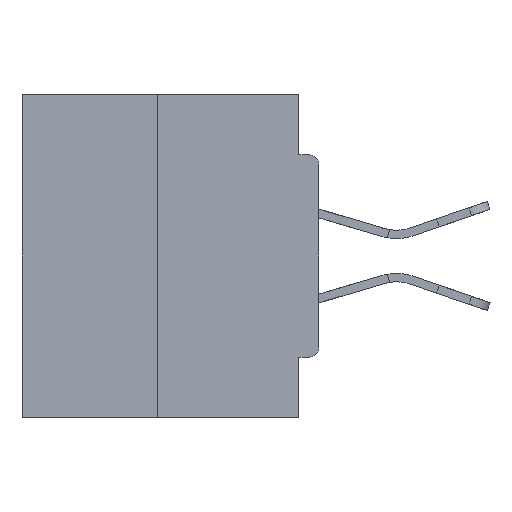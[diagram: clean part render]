
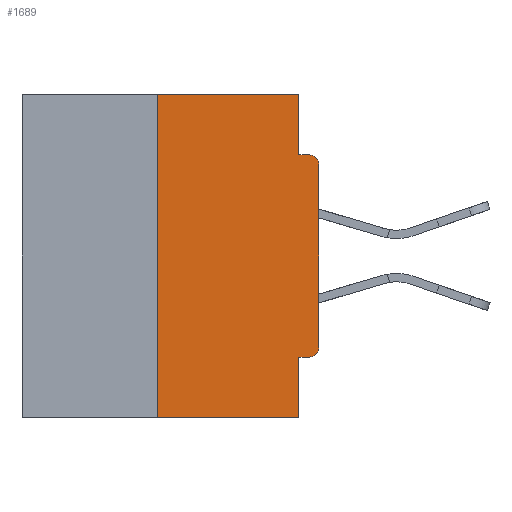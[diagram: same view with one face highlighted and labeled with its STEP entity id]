
A CAD part, left-side view. The second image highlights one B-rep face of the part: STEP entity #1689.
In plain terms, the highlighted planar face has unit normal (-1, 0, 0).
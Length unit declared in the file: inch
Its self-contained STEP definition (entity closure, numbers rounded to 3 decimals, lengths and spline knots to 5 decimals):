
#196 = CARTESIAN_POINT ( 'NONE',  ( 0., 0.031, 0. ) ) ;
#494 = DIRECTION ( 'NONE',  ( 0., 0., 1. ) ) ;
#618 = LINE ( 'NONE', #21622, #19033 ) ;
#691 = VECTOR ( 'NONE', #16077, 39.37008 ) ;
#942 = VERTEX_POINT ( 'NONE', #22931 ) ;
#1689 = ADVANCED_FACE ( 'NONE', ( #21442 ), #31949, .F. ) ;
#1726 = LINE ( 'NONE', #17066, #4128 ) ;
#1765 = AXIS2_PLACEMENT_3D ( 'NONE', #20414, #2351, #12517 ) ;
#2313 = LINE ( 'NONE', #7808, #17178 ) ;
#2351 = DIRECTION ( 'NONE',  ( -1., 0., 0. ) ) ;
#2788 = CARTESIAN_POINT ( 'NONE',  ( 0., 0.015, -0.1085 ) ) ;
#3073 = LINE ( 'NONE', #11176, #21508 ) ;
#3281 = ORIENTED_EDGE ( 'NONE', *, *, #24831, .F. ) ;
#3482 = EDGE_LOOP ( 'NONE', ( #13902, #20780, #18698, #6443, #3281, #6612, #5165, #19650, #14444, #18623 ) ) ;
#3980 = CIRCLE ( 'NONE', #1765, 0.015 ) ;
#4121 = AXIS2_PLACEMENT_3D ( 'NONE', #23693, #24210, #31613 ) ;
#4128 = VECTOR ( 'NONE', #17236, 39.37008 ) ;
#4614 = EDGE_CURVE ( 'NONE', #7501, #12881, #1726, .T. ) ;
#4725 = DIRECTION ( 'NONE',  ( 0., -1., 0. ) ) ;
#4865 = VERTEX_POINT ( 'NONE', #29097 ) ;
#5165 = ORIENTED_EDGE ( 'NONE', *, *, #24865, .T. ) ;
#5357 = LINE ( 'NONE', #196, #16672 ) ;
#6097 = AXIS2_PLACEMENT_3D ( 'NONE', #2788, #28809, #24151 ) ;
#6355 = VERTEX_POINT ( 'NONE', #22722 ) ;
#6443 = ORIENTED_EDGE ( 'NONE', *, *, #21033, .F. ) ;
#6612 = ORIENTED_EDGE ( 'NONE', *, *, #31259, .T. ) ;
#6807 = DIRECTION ( 'NONE',  ( 0., 0., 1. ) ) ;
#7501 = VERTEX_POINT ( 'NONE', #8539 ) ;
#7808 = CARTESIAN_POINT ( 'NONE',  ( 0., 0., -0.0935 ) ) ;
#8313 = VERTEX_POINT ( 'NONE', #21533 ) ;
#8539 = CARTESIAN_POINT ( 'NONE',  ( 0., 0.25, -0.5 ) ) ;
#9038 = VECTOR ( 'NONE', #4725, 39.37008 ) ;
#11176 = CARTESIAN_POINT ( 'NONE',  ( 0., 0.25, 0. ) ) ;
#12140 = CARTESIAN_POINT ( 'NONE',  ( 0., 0., 0. ) ) ;
#12517 = DIRECTION ( 'NONE',  ( 0., 0., -1. ) ) ;
#12656 = DIRECTION ( 'NONE',  ( 0., -1., 0. ) ) ;
#12881 = VERTEX_POINT ( 'NONE', #23540 ) ;
#13530 = CARTESIAN_POINT ( 'NONE',  ( 0., 0.25, 0. ) ) ;
#13902 = ORIENTED_EDGE ( 'NONE', *, *, #15880, .F. ) ;
#14444 = ORIENTED_EDGE ( 'NONE', *, *, #32921, .F. ) ;
#15473 = CIRCLE ( 'NONE', #6097, 0.015 ) ;
#15880 = EDGE_CURVE ( 'NONE', #31340, #4865, #31394, .T. ) ;
#16077 = DIRECTION ( 'NONE',  ( 0., 0., -1. ) ) ;
#16415 = CARTESIAN_POINT ( 'NONE',  ( 0., 0.031, -0.5 ) ) ;
#16672 = VECTOR ( 'NONE', #26536, 39.37008 ) ;
#17066 = CARTESIAN_POINT ( 'NONE',  ( 0., 0.46, -0.5 ) ) ;
#17178 = VECTOR ( 'NONE', #12656, 39.37008 ) ;
#17236 = DIRECTION ( 'NONE',  ( 0., -1., 0. ) ) ;
#17933 = CARTESIAN_POINT ( 'NONE',  ( 0., 0.031, -0.4065 ) ) ;
#18623 = ORIENTED_EDGE ( 'NONE', *, *, #33701, .F. ) ;
#18698 = ORIENTED_EDGE ( 'NONE', *, *, #4614, .T. ) ;
#19033 = VECTOR ( 'NONE', #30394, 39.37008 ) ;
#19650 = ORIENTED_EDGE ( 'NONE', *, *, #19755, .T. ) ;
#19755 = EDGE_CURVE ( 'NONE', #6355, #8313, #15473, .T. ) ;
#20414 = CARTESIAN_POINT ( 'NONE',  ( 0., 0.015, -0.3915 ) ) ;
#20780 = ORIENTED_EDGE ( 'NONE', *, *, #32224, .F. ) ;
#21033 = EDGE_CURVE ( 'NONE', #25628, #12881, #26392, .T. ) ;
#21442 = FACE_OUTER_BOUND ( 'NONE', #3482, .T. ) ;
#21508 = VECTOR ( 'NONE', #494, 39.37008 ) ;
#21533 = CARTESIAN_POINT ( 'NONE',  ( 0., 0.015, -0.0935 ) ) ;
#21622 = CARTESIAN_POINT ( 'NONE',  ( 0., 0., -0.4065 ) ) ;
#22722 = CARTESIAN_POINT ( 'NONE',  ( 0., 0., -0.1085 ) ) ;
#22931 = CARTESIAN_POINT ( 'NONE',  ( 0., 0.015, -0.4065 ) ) ;
#23395 = VERTEX_POINT ( 'NONE', #24756 ) ;
#23540 = CARTESIAN_POINT ( 'NONE',  ( 0., 0.031, -0.5 ) ) ;
#23693 = CARTESIAN_POINT ( 'NONE',  ( 0., 0.46, 0. ) ) ;
#24151 = DIRECTION ( 'NONE',  ( 0., 0., -1. ) ) ;
#24210 = DIRECTION ( 'NONE',  ( 1., 0., 0. ) ) ;
#24756 = CARTESIAN_POINT ( 'NONE',  ( 0., 0., -0.3915 ) ) ;
#24831 = EDGE_CURVE ( 'NONE', #942, #25628, #618, .T. ) ;
#24865 = EDGE_CURVE ( 'NONE', #23395, #6355, #25058, .T. ) ;
#25058 = LINE ( 'NONE', #12140, #25658 ) ;
#25628 = VERTEX_POINT ( 'NONE', #17933 ) ;
#25658 = VECTOR ( 'NONE', #6807, 39.37008 ) ;
#26392 = LINE ( 'NONE', #16415, #691 ) ;
#26475 = VERTEX_POINT ( 'NONE', #31232 ) ;
#26536 = DIRECTION ( 'NONE',  ( 0., 0., -1. ) ) ;
#28311 = CARTESIAN_POINT ( 'NONE',  ( 0., 0.46, 0. ) ) ;
#28809 = DIRECTION ( 'NONE',  ( -1., 0., 0. ) ) ;
#29097 = CARTESIAN_POINT ( 'NONE',  ( 0., 0.031, 0. ) ) ;
#30394 = DIRECTION ( 'NONE',  ( 0., 1., 0. ) ) ;
#31232 = CARTESIAN_POINT ( 'NONE',  ( 0., 0.031, -0.0935 ) ) ;
#31259 = EDGE_CURVE ( 'NONE', #942, #23395, #3980, .T. ) ;
#31340 = VERTEX_POINT ( 'NONE', #13530 ) ;
#31394 = LINE ( 'NONE', #28311, #9038 ) ;
#31613 = DIRECTION ( 'NONE',  ( 0., 0., -1. ) ) ;
#31949 = PLANE ( 'NONE',  #4121 ) ;
#32224 = EDGE_CURVE ( 'NONE', #7501, #31340, #3073, .T. ) ;
#32921 = EDGE_CURVE ( 'NONE', #26475, #8313, #2313, .T. ) ;
#33701 = EDGE_CURVE ( 'NONE', #4865, #26475, #5357, .T. ) ;
